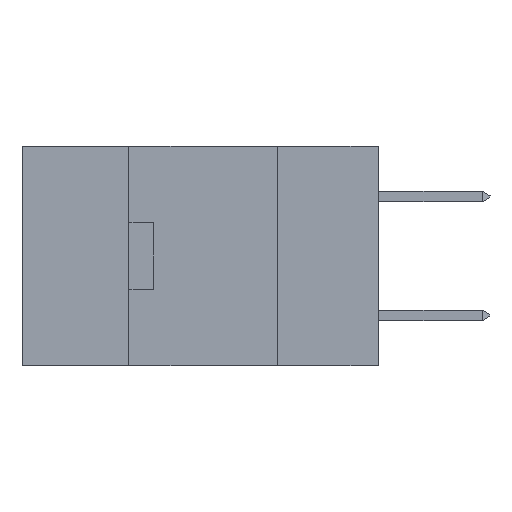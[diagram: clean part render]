
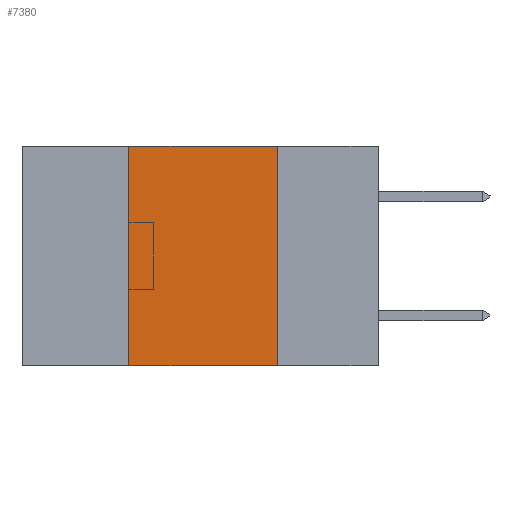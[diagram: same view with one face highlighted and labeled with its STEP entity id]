
A CAD part, left-side view. The second image highlights one B-rep face of the part: STEP entity #7380.
In plain terms, the highlighted planar face has unit normal (-1, 0, 0).
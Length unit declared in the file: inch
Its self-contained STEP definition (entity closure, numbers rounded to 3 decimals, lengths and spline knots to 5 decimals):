
#971 = LINE ( 'NONE', #24643, #24769 ) ;
#1823 = DIRECTION ( 'NONE',  ( 0., 0., 1. ) ) ;
#2205 = DIRECTION ( 'NONE',  ( 0., 0., -1. ) ) ;
#2981 = DIRECTION ( 'NONE',  ( 1., 0., 0. ) ) ;
#3595 = ORIENTED_EDGE ( 'NONE', *, *, #23933, .T. ) ;
#3614 = EDGE_CURVE ( 'NONE', #19840, #12355, #971, .T. ) ;
#4958 = DIRECTION ( 'NONE',  ( 0., 0., -1. ) ) ;
#5083 = LINE ( 'NONE', #25046, #18181 ) ;
#5100 = PLANE ( 'NONE',  #25332 ) ;
#5843 = VERTEX_POINT ( 'NONE', #24069 ) ;
#7380 = ADVANCED_FACE ( 'NONE', ( #9203 ), #5100, .F. ) ;
#8204 = CARTESIAN_POINT ( 'NONE',  ( 0., 0.17, 0. ) ) ;
#9203 = FACE_OUTER_BOUND ( 'NONE', #22613, .T. ) ;
#9732 = CARTESIAN_POINT ( 'NONE',  ( 0., 0.42, 0. ) ) ;
#10467 = CARTESIAN_POINT ( 'NONE',  ( 0., 0.42, -0.37 ) ) ;
#10713 = LINE ( 'NONE', #23726, #26221 ) ;
#11742 = VECTOR ( 'NONE', #1823, 39.37008 ) ;
#12355 = VERTEX_POINT ( 'NONE', #8204 ) ;
#12603 = LINE ( 'NONE', #10467, #11742 ) ;
#17379 = VERTEX_POINT ( 'NONE', #27343 ) ;
#17431 = ORIENTED_EDGE ( 'NONE', *, *, #21427, .F. ) ;
#18181 = VECTOR ( 'NONE', #22216, 39.37008 ) ;
#18418 = DIRECTION ( 'NONE',  ( 0., -1., 0. ) ) ;
#19840 = VERTEX_POINT ( 'NONE', #9732 ) ;
#19993 = EDGE_CURVE ( 'NONE', #12355, #5843, #10713, .T. ) ;
#21427 = EDGE_CURVE ( 'NONE', #17379, #19840, #12603, .T. ) ;
#22216 = DIRECTION ( 'NONE',  ( 0., -1., 0. ) ) ;
#22613 = EDGE_LOOP ( 'NONE', ( #27432, #26639, #17431, #3595 ) ) ;
#23726 = CARTESIAN_POINT ( 'NONE',  ( 0., 0.17, -0.37 ) ) ;
#23933 = EDGE_CURVE ( 'NONE', #17379, #5843, #5083, .T. ) ;
#24069 = CARTESIAN_POINT ( 'NONE',  ( 0., 0.17, -0.37 ) ) ;
#24643 = CARTESIAN_POINT ( 'NONE',  ( 0., 0.6, 0. ) ) ;
#24769 = VECTOR ( 'NONE', #18418, 39.37008 ) ;
#24780 = CARTESIAN_POINT ( 'NONE',  ( 0., 0.6, 0. ) ) ;
#25046 = CARTESIAN_POINT ( 'NONE',  ( 0., 0.6, -0.37 ) ) ;
#25332 = AXIS2_PLACEMENT_3D ( 'NONE', #24780, #2981, #4958 ) ;
#26221 = VECTOR ( 'NONE', #2205, 39.37008 ) ;
#26639 = ORIENTED_EDGE ( 'NONE', *, *, #3614, .F. ) ;
#27343 = CARTESIAN_POINT ( 'NONE',  ( 0., 0.42, -0.37 ) ) ;
#27432 = ORIENTED_EDGE ( 'NONE', *, *, #19993, .F. ) ;
